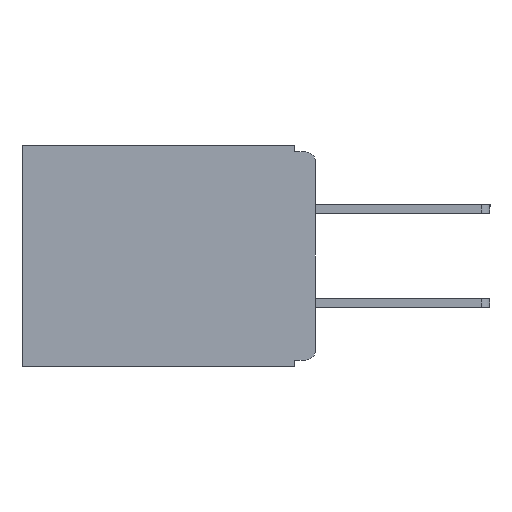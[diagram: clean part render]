
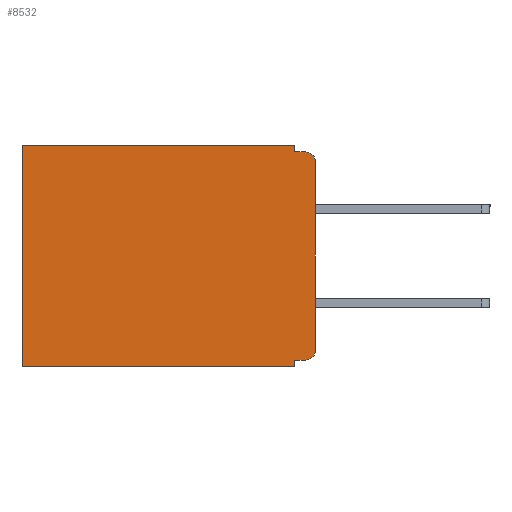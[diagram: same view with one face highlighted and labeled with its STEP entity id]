
A CAD part, left-side view. The second image highlights one B-rep face of the part: STEP entity #8532.
In plain terms, the highlighted planar face has unit normal (-1, 0, 0).
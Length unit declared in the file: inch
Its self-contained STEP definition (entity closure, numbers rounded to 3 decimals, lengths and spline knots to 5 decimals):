
#121 = CARTESIAN_POINT ( 'NONE',  ( 0.3, 0.015, -0.01 ) ) ;
#276 = DIRECTION ( 'NONE',  ( 0., 0., -1. ) ) ;
#558 = DIRECTION ( 'NONE',  ( 0., -1., 0. ) ) ;
#594 = ORIENTED_EDGE ( 'NONE', *, *, #20335, .F. ) ;
#892 = CARTESIAN_POINT ( 'NONE',  ( 0.3, 0.031, 0. ) ) ;
#1035 = CARTESIAN_POINT ( 'NONE',  ( 0.3, 0.031, -0.33 ) ) ;
#2031 = VERTEX_POINT ( 'NONE', #5542 ) ;
#2122 = VERTEX_POINT ( 'NONE', #121 ) ;
#3309 = VERTEX_POINT ( 'NONE', #1035 ) ;
#4040 = DIRECTION ( 'NONE',  ( 0., 1., 0. ) ) ;
#4080 = VERTEX_POINT ( 'NONE', #16404 ) ;
#4760 = EDGE_CURVE ( 'NONE', #30249, #15890, #28776, .T. ) ;
#4974 = DIRECTION ( 'NONE',  ( -1., 0., 0. ) ) ;
#5026 = VECTOR ( 'NONE', #17998, 39.37008 ) ;
#5542 = CARTESIAN_POINT ( 'NONE',  ( 0.3, 0.437, 0. ) ) ;
#5843 = LINE ( 'NONE', #33746, #5026 ) ;
#6574 = PLANE ( 'NONE',  #10134 ) ;
#6824 = LINE ( 'NONE', #17355, #34123 ) ;
#6934 = CARTESIAN_POINT ( 'NONE',  ( 0.3, 0.031, 0. ) ) ;
#8154 = EDGE_CURVE ( 'NONE', #2031, #20769, #5843, .T. ) ;
#8532 = ADVANCED_FACE ( 'NONE', ( #30291 ), #6574, .F. ) ;
#8758 = CARTESIAN_POINT ( 'NONE',  ( 0.3, 0., -0.33 ) ) ;
#8970 = VECTOR ( 'NONE', #27361, 39.37008 ) ;
#9269 = DIRECTION ( 'NONE',  ( 1., 0., 0. ) ) ;
#9283 = ORIENTED_EDGE ( 'NONE', *, *, #21336, .F. ) ;
#10134 = AXIS2_PLACEMENT_3D ( 'NONE', #25111, #9269, #27788 ) ;
#10207 = EDGE_CURVE ( 'NONE', #15890, #2122, #11568, .T. ) ;
#10290 = DIRECTION ( 'NONE',  ( 0., 1., 0. ) ) ;
#10594 = ORIENTED_EDGE ( 'NONE', *, *, #22483, .T. ) ;
#10649 = CARTESIAN_POINT ( 'NONE',  ( 0.3, 0.015, -0.32 ) ) ;
#10687 = VERTEX_POINT ( 'NONE', #10649 ) ;
#10976 = VECTOR ( 'NONE', #10290, 39.37008 ) ;
#11568 = LINE ( 'NONE', #19286, #31827 ) ;
#12977 = ORIENTED_EDGE ( 'NONE', *, *, #21511, .F. ) ;
#13503 = CARTESIAN_POINT ( 'NONE',  ( 0.3, 0.015, -0.025 ) ) ;
#13521 = VERTEX_POINT ( 'NONE', #26440 ) ;
#13894 = VECTOR ( 'NONE', #34364, 39.37008 ) ;
#13906 = LINE ( 'NONE', #8758, #20962 ) ;
#15890 = VERTEX_POINT ( 'NONE', #29548 ) ;
#16150 = DIRECTION ( 'NONE',  ( 0., 0., -1. ) ) ;
#16404 = CARTESIAN_POINT ( 'NONE',  ( 0.3, 0.031, -0.32 ) ) ;
#17226 = CIRCLE ( 'NONE', #22829, 0.015 ) ;
#17355 = CARTESIAN_POINT ( 'NONE',  ( 0.3, 0., 0. ) ) ;
#17998 = DIRECTION ( 'NONE',  ( 0., 0., -1. ) ) ;
#18070 = LINE ( 'NONE', #33958, #10976 ) ;
#18112 = EDGE_LOOP ( 'NONE', ( #33544, #32105, #31687, #21141, #31879, #27238, #9283, #12977, #594, #10594 ) ) ;
#18497 = CARTESIAN_POINT ( 'NONE',  ( 0.3, 0.437, -0.33 ) ) ;
#19286 = CARTESIAN_POINT ( 'NONE',  ( 0.3, 0., -0.01 ) ) ;
#20335 = EDGE_CURVE ( 'NONE', #10687, #4080, #27617, .T. ) ;
#20480 = AXIS2_PLACEMENT_3D ( 'NONE', #20929, #4974, #23528 ) ;
#20769 = VERTEX_POINT ( 'NONE', #18497 ) ;
#20929 = CARTESIAN_POINT ( 'NONE',  ( 0.3, 0.015, -0.305 ) ) ;
#20962 = VECTOR ( 'NONE', #24621, 39.37008 ) ;
#21141 = ORIENTED_EDGE ( 'NONE', *, *, #4760, .F. ) ;
#21336 = EDGE_CURVE ( 'NONE', #3309, #20769, #18070, .T. ) ;
#21511 = EDGE_CURVE ( 'NONE', #4080, #3309, #34098, .T. ) ;
#22057 = CARTESIAN_POINT ( 'NONE',  ( 0.3, 0., -0.32 ) ) ;
#22483 = EDGE_CURVE ( 'NONE', #10687, #13521, #23382, .T. ) ;
#22829 = AXIS2_PLACEMENT_3D ( 'NONE', #13503, #31972, #16150 ) ;
#23382 = CIRCLE ( 'NONE', #20480, 0.015 ) ;
#23528 = DIRECTION ( 'NONE',  ( 0., 0., -1. ) ) ;
#24621 = DIRECTION ( 'NONE',  ( 0., 0., -1. ) ) ;
#25111 = CARTESIAN_POINT ( 'NONE',  ( 0.3, 0., -0.33 ) ) ;
#26440 = CARTESIAN_POINT ( 'NONE',  ( 0.3, 0., -0.305 ) ) ;
#27238 = ORIENTED_EDGE ( 'NONE', *, *, #8154, .T. ) ;
#27361 = DIRECTION ( 'NONE',  ( 0., 1., 0. ) ) ;
#27617 = LINE ( 'NONE', #22057, #8970 ) ;
#27788 = DIRECTION ( 'NONE',  ( 0., 0., -1. ) ) ;
#28136 = VERTEX_POINT ( 'NONE', #33630 ) ;
#28776 = LINE ( 'NONE', #892, #13894 ) ;
#29548 = CARTESIAN_POINT ( 'NONE',  ( 0.3, 0.031, -0.01 ) ) ;
#29554 = EDGE_CURVE ( 'NONE', #30249, #2031, #6824, .T. ) ;
#29899 = EDGE_CURVE ( 'NONE', #28136, #2122, #17226, .T. ) ;
#30249 = VERTEX_POINT ( 'NONE', #6934 ) ;
#30291 = FACE_OUTER_BOUND ( 'NONE', #18112, .T. ) ;
#31687 = ORIENTED_EDGE ( 'NONE', *, *, #10207, .F. ) ;
#31827 = VECTOR ( 'NONE', #558, 39.37008 ) ;
#31879 = ORIENTED_EDGE ( 'NONE', *, *, #29554, .T. ) ;
#31972 = DIRECTION ( 'NONE',  ( -1., 0., 0. ) ) ;
#32002 = EDGE_CURVE ( 'NONE', #28136, #13521, #13906, .T. ) ;
#32105 = ORIENTED_EDGE ( 'NONE', *, *, #29899, .T. ) ;
#32125 = CARTESIAN_POINT ( 'NONE',  ( 0.3, 0.031, -0.33 ) ) ;
#33279 = VECTOR ( 'NONE', #276, 39.37008 ) ;
#33544 = ORIENTED_EDGE ( 'NONE', *, *, #32002, .F. ) ;
#33630 = CARTESIAN_POINT ( 'NONE',  ( 0.3, 0., -0.025 ) ) ;
#33746 = CARTESIAN_POINT ( 'NONE',  ( 0.3, 0.437, -0.33 ) ) ;
#33958 = CARTESIAN_POINT ( 'NONE',  ( 0.3, 0., -0.33 ) ) ;
#34098 = LINE ( 'NONE', #32125, #33279 ) ;
#34123 = VECTOR ( 'NONE', #4040, 39.37008 ) ;
#34364 = DIRECTION ( 'NONE',  ( 0., 0., -1. ) ) ;
